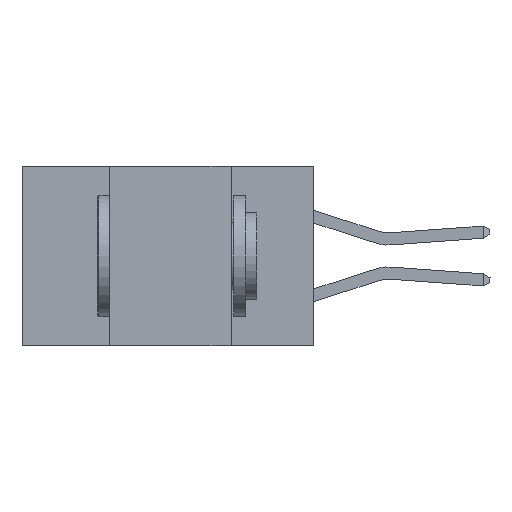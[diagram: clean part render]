
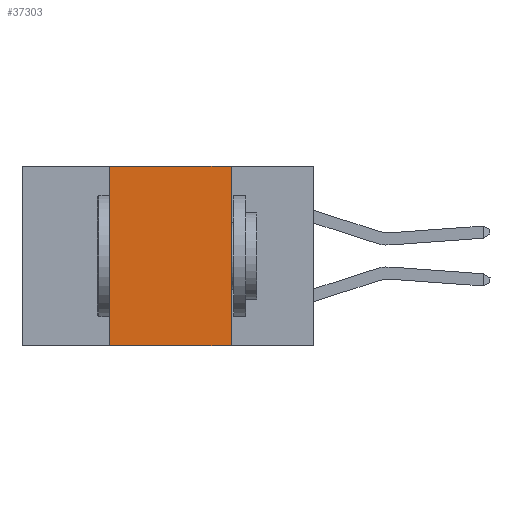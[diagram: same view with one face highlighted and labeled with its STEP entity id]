
A CAD part, left-side view. The second image highlights one B-rep face of the part: STEP entity #37303.
In plain terms, the highlighted planar face has unit normal (-1, 0, 0).
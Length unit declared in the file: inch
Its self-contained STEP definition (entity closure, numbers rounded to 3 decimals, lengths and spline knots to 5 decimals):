
#43 = ORIENTED_EDGE ( 'NONE', *, *, #14532, .F. ) ;
#2205 = CARTESIAN_POINT ( 'NONE',  ( 0., 0.6, -0.37 ) ) ;
#3019 = EDGE_CURVE ( 'NONE', #6495, #39502, #16259, .T. ) ;
#6495 = VERTEX_POINT ( 'NONE', #12385 ) ;
#7544 = FACE_OUTER_BOUND ( 'NONE', #34966, .T. ) ;
#9506 = PLANE ( 'NONE',  #19437 ) ;
#9780 = CARTESIAN_POINT ( 'NONE',  ( 0., 0.6, 0. ) ) ;
#9788 = CARTESIAN_POINT ( 'NONE',  ( 0., 0.6, 0. ) ) ;
#11475 = CARTESIAN_POINT ( 'NONE',  ( 0., 0.17, -0.37 ) ) ;
#12385 = CARTESIAN_POINT ( 'NONE',  ( 0., 0.42, 0. ) ) ;
#12696 = DIRECTION ( 'NONE',  ( 0., 0., -1. ) ) ;
#13331 = ORIENTED_EDGE ( 'NONE', *, *, #28428, .T. ) ;
#14496 = EDGE_CURVE ( 'NONE', #24784, #6495, #36215, .T. ) ;
#14532 = EDGE_CURVE ( 'NONE', #39502, #34892, #27760, .T. ) ;
#14897 = VECTOR ( 'NONE', #40684, 39.37008 ) ;
#15113 = ORIENTED_EDGE ( 'NONE', *, *, #3019, .F. ) ;
#16259 = LINE ( 'NONE', #9780, #35106 ) ;
#18413 = LINE ( 'NONE', #2205, #23840 ) ;
#18502 = DIRECTION ( 'NONE',  ( 0., 0., 1. ) ) ;
#19437 = AXIS2_PLACEMENT_3D ( 'NONE', #9788, #31649, #12696 ) ;
#23840 = VECTOR ( 'NONE', #30681, 39.37008 ) ;
#24481 = CARTESIAN_POINT ( 'NONE',  ( 0., 0.17, 0. ) ) ;
#24784 = VERTEX_POINT ( 'NONE', #40440 ) ;
#24868 = CARTESIAN_POINT ( 'NONE',  ( 0., 0.17, 0. ) ) ;
#27760 = LINE ( 'NONE', #24868, #14897 ) ;
#27765 = CARTESIAN_POINT ( 'NONE',  ( 0., 0.42, 0. ) ) ;
#28428 = EDGE_CURVE ( 'NONE', #24784, #34892, #18413, .T. ) ;
#29274 = VECTOR ( 'NONE', #18502, 39.37008 ) ;
#30681 = DIRECTION ( 'NONE',  ( 0., -1., 0. ) ) ;
#31649 = DIRECTION ( 'NONE',  ( 1., 0., 0. ) ) ;
#31925 = DIRECTION ( 'NONE',  ( 0., -1., 0. ) ) ;
#34892 = VERTEX_POINT ( 'NONE', #11475 ) ;
#34966 = EDGE_LOOP ( 'NONE', ( #43, #15113, #35761, #13331 ) ) ;
#35106 = VECTOR ( 'NONE', #31925, 39.37008 ) ;
#35761 = ORIENTED_EDGE ( 'NONE', *, *, #14496, .F. ) ;
#36215 = LINE ( 'NONE', #27765, #29274 ) ;
#37303 = ADVANCED_FACE ( 'NONE', ( #7544 ), #9506, .F. ) ;
#39502 = VERTEX_POINT ( 'NONE', #24481 ) ;
#40440 = CARTESIAN_POINT ( 'NONE',  ( 0., 0.42, -0.37 ) ) ;
#40684 = DIRECTION ( 'NONE',  ( 0., 0., -1. ) ) ;
